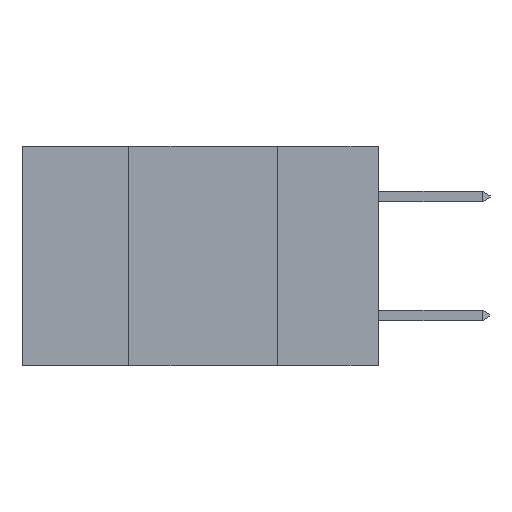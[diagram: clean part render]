
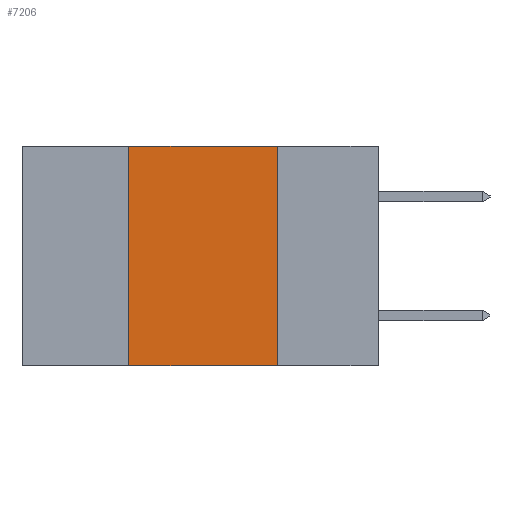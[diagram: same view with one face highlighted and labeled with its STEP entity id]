
A CAD part, left-side view. The second image highlights one B-rep face of the part: STEP entity #7206.
In plain terms, the highlighted planar face has unit normal (-1, 0, 0).
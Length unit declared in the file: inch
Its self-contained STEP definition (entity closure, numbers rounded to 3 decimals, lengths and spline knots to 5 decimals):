
#359 = CARTESIAN_POINT ( 'NONE',  ( 0., 0.6, 0. ) ) ;
#463 = AXIS2_PLACEMENT_3D ( 'NONE', #359, #11003, #2417 ) ;
#940 = CARTESIAN_POINT ( 'NONE',  ( 0., 0.42, 0. ) ) ;
#984 = CARTESIAN_POINT ( 'NONE',  ( 0., 0.42, -0.37 ) ) ;
#1292 = VERTEX_POINT ( 'NONE', #10393 ) ;
#1355 = PLANE ( 'NONE',  #463 ) ;
#1483 = EDGE_CURVE ( 'NONE', #10754, #1292, #3516, .T. ) ;
#1559 = EDGE_CURVE ( 'NONE', #1292, #3972, #6072, .T. ) ;
#2417 = DIRECTION ( 'NONE',  ( 0., 0., -1. ) ) ;
#2429 = DIRECTION ( 'NONE',  ( 0., 0., -1. ) ) ;
#3516 = LINE ( 'NONE', #12242, #7891 ) ;
#3972 = VERTEX_POINT ( 'NONE', #9240 ) ;
#4625 = CARTESIAN_POINT ( 'NONE',  ( 0., 0.6, -0.37 ) ) ;
#4764 = DIRECTION ( 'NONE',  ( 0., 0., 1. ) ) ;
#5464 = VERTEX_POINT ( 'NONE', #11973 ) ;
#5615 = ORIENTED_EDGE ( 'NONE', *, *, #1559, .F. ) ;
#6031 = EDGE_CURVE ( 'NONE', #5464, #3972, #11230, .T. ) ;
#6072 = LINE ( 'NONE', #11012, #7504 ) ;
#6582 = ORIENTED_EDGE ( 'NONE', *, *, #1483, .F. ) ;
#7206 = ADVANCED_FACE ( 'NONE', ( #8192 ), #1355, .F. ) ;
#7321 = VECTOR ( 'NONE', #10470, 39.37008 ) ;
#7504 = VECTOR ( 'NONE', #2429, 39.37008 ) ;
#7891 = VECTOR ( 'NONE', #12312, 39.37008 ) ;
#8192 = FACE_OUTER_BOUND ( 'NONE', #8855, .T. ) ;
#8249 = EDGE_CURVE ( 'NONE', #5464, #10754, #9570, .T. ) ;
#8368 = ORIENTED_EDGE ( 'NONE', *, *, #8249, .F. ) ;
#8855 = EDGE_LOOP ( 'NONE', ( #5615, #6582, #8368, #12193 ) ) ;
#9240 = CARTESIAN_POINT ( 'NONE',  ( 0., 0.17, -0.37 ) ) ;
#9570 = LINE ( 'NONE', #984, #10609 ) ;
#10393 = CARTESIAN_POINT ( 'NONE',  ( 0., 0.17, 0. ) ) ;
#10470 = DIRECTION ( 'NONE',  ( 0., -1., 0. ) ) ;
#10609 = VECTOR ( 'NONE', #4764, 39.37008 ) ;
#10754 = VERTEX_POINT ( 'NONE', #940 ) ;
#11003 = DIRECTION ( 'NONE',  ( 1., 0., 0. ) ) ;
#11012 = CARTESIAN_POINT ( 'NONE',  ( 0., 0.17, -0.37 ) ) ;
#11230 = LINE ( 'NONE', #4625, #7321 ) ;
#11973 = CARTESIAN_POINT ( 'NONE',  ( 0., 0.42, -0.37 ) ) ;
#12193 = ORIENTED_EDGE ( 'NONE', *, *, #6031, .T. ) ;
#12242 = CARTESIAN_POINT ( 'NONE',  ( 0., 0.6, 0. ) ) ;
#12312 = DIRECTION ( 'NONE',  ( 0., -1., 0. ) ) ;
